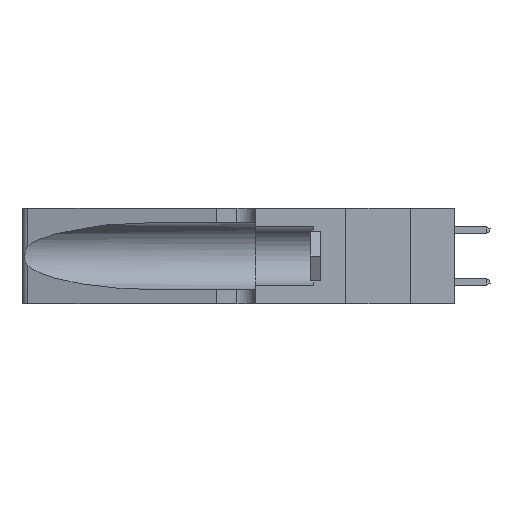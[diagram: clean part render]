
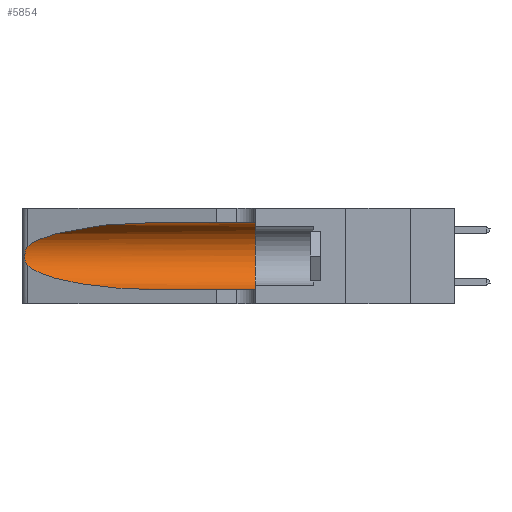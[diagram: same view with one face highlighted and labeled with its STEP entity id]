
A CAD part, left-side view. The second image highlights one B-rep face of the part: STEP entity #5854.
In plain terms, the highlighted cylindrical face has radius 3.308 mm (diameter 6.617 mm), a partial arc.
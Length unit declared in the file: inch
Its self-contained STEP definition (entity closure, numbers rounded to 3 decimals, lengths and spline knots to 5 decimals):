
#1498 = DIRECTION ( 'NONE',  ( 0., 0., -1. ) ) ;
#1572 = DIRECTION ( 'NONE',  ( 0., -1., 0. ) ) ;
#1588 = DIRECTION ( 'NONE',  ( 0., -1., 0. ) ) ;
#1725 = AXIS2_PLACEMENT_3D ( 'NONE', #24249, #1588, #1498 ) ;
#2300 =( BOUNDED_CURVE ( )  B_SPLINE_CURVE ( 3, ( #16898, #26721, #22228, #10949 ),
 .UNSPECIFIED., .F., .T. ) 
 B_SPLINE_CURVE_WITH_KNOTS ( ( 4, 4 ),
 ( 3.44316, 4.71239 ),
 .UNSPECIFIED. ) 
 CURVE ( )  GEOMETRIC_REPRESENTATION_ITEM ( )  RATIONAL_B_SPLINE_CURVE ( ( 1., 0.87, 0.87, 1. ) ) 
 REPRESENTATION_ITEM ( '' )  );
#2474 = CYLINDRICAL_SURFACE ( 'NONE', #1725, 0.13025 ) ;
#4036 = LINE ( 'NONE', #24258, #20734 ) ;
#4125 = CARTESIAN_POINT ( 'NONE',  ( 0.25487, 1.22718, 0.14631 ) ) ;
#4606 = CARTESIAN_POINT ( 'NONE',  ( 0.25639, 1.23184, 0.21858 ) ) ;
#5854 = ADVANCED_FACE ( 'NONE', ( #7828 ), #2474, .F. ) ;
#6089 = CARTESIAN_POINT ( 'NONE',  ( 0.26075, 1.23896, 0.19203 ) ) ;
#6331 = CARTESIAN_POINT ( 'NONE',  ( 0.26075, 1.23896, 0.178 ) ) ;
#7218 = CARTESIAN_POINT ( 'NONE',  ( 0.1305, 0.35, 0.185 ) ) ;
#7424 = ORIENTED_EDGE ( 'NONE', *, *, #10110, .T. ) ;
#7828 = FACE_OUTER_BOUND ( 'NONE', #10877, .T. ) ;
#8082 = EDGE_CURVE ( 'NONE', #15675, #22160, #2300, .T. ) ;
#8282 = CARTESIAN_POINT ( 'NONE',  ( 0.25854, 1.2359, 0.20912 ) ) ;
#8344 = CARTESIAN_POINT ( 'NONE',  ( 0.1305, 1.61858, 0.05475 ) ) ;
#9031 = CARTESIAN_POINT ( 'NONE',  ( 0.1305, 0.72297, 0.31525 ) ) ;
#10110 = EDGE_CURVE ( 'NONE', #22160, #10908, #26794, .T. ) ;
#10643 = CARTESIAN_POINT ( 'NONE',  ( 0.2373, 1.15595, 0.28018 ) ) ;
#10764 = VERTEX_POINT ( 'NONE', #26175 ) ;
#10877 = EDGE_LOOP ( 'NONE', ( #24536, #21921, #24334, #7424, #19852, #14446 ) ) ;
#10908 = VERTEX_POINT ( 'NONE', #22279 ) ;
#10949 = CARTESIAN_POINT ( 'NONE',  ( 0.1305, 0.72297, 0.05475 ) ) ;
#11233 = CARTESIAN_POINT ( 'NONE',  ( 0.25787, 1.23484, 0.2124 ) ) ;
#11376 = EDGE_CURVE ( 'NONE', #24390, #26412, #4036, .T. ) ;
#12306 = CARTESIAN_POINT ( 'NONE',  ( 0.25487, 1.22718, 0.22369 ) ) ;
#13304 = CARTESIAN_POINT ( 'NONE',  ( 0.25639, 1.23186, 0.15144 ) ) ;
#14188 = CIRCLE ( 'NONE', #24427, 0.13025 ) ;
#14346 = CARTESIAN_POINT ( 'NONE',  ( 0.25555, 1.22994, 0.2215 ) ) ;
#14396 = CARTESIAN_POINT ( 'NONE',  ( 0.26018, 1.23835, 0.19895 ) ) ;
#14424 = EDGE_CURVE ( 'NONE', #26412, #10908, #14188, .T. ) ;
#14446 = ORIENTED_EDGE ( 'NONE', *, *, #11376, .F. ) ;
#14663 = CARTESIAN_POINT ( 'NONE',  ( 0.25487, 1.22718, 0.14631 ) ) ;
#15481 = CARTESIAN_POINT ( 'NONE',  ( 0.26017, 1.23833, 0.17102 ) ) ;
#15489 = CARTESIAN_POINT ( 'NONE',  ( 0.1305, 0.72297, 0.05475 ) ) ;
#15575 = CARTESIAN_POINT ( 'NONE',  ( 0.25555, 1.22993, 0.14849 ) ) ;
#15675 = VERTEX_POINT ( 'NONE', #14663 ) ;
#15971 = EDGE_CURVE ( 'NONE', #10764, #15675, #27092, .T. ) ;
#16898 = CARTESIAN_POINT ( 'NONE',  ( 0.25487, 1.22718, 0.14631 ) ) ;
#17642 = CARTESIAN_POINT ( 'NONE',  ( 0.1305, 0.35, 0.31525 ) ) ;
#17746 = CARTESIAN_POINT ( 'NONE',  ( 0.25856, 1.23593, 0.16098 ) ) ;
#18058 = CARTESIAN_POINT ( 'NONE',  ( 0.18966, 0.96281, 0.31525 ) ) ;
#19852 = ORIENTED_EDGE ( 'NONE', *, *, #14424, .F. ) ;
#20734 = VECTOR ( 'NONE', #21660, 39.37008 ) ;
#20750 = VECTOR ( 'NONE', #1572, 39.37008 ) ;
#20777 = EDGE_CURVE ( 'NONE', #24390, #10764, #21792, .T. ) ;
#21096 = DIRECTION ( 'NONE',  ( 0., 0., 1. ) ) ;
#21660 = DIRECTION ( 'NONE',  ( 0., -1., 0. ) ) ;
#21792 =( BOUNDED_CURVE ( )  B_SPLINE_CURVE ( 3, ( #9031, #18058, #10643, #22311 ),
 .UNSPECIFIED., .F., .T. ) 
 B_SPLINE_CURVE_WITH_KNOTS ( ( 4, 4 ),
 ( 1.5708, 2.84003 ),
 .UNSPECIFIED. ) 
 CURVE ( )  GEOMETRIC_REPRESENTATION_ITEM ( )  RATIONAL_B_SPLINE_CURVE ( ( 1., 0.87, 0.87, 1. ) ) 
 REPRESENTATION_ITEM ( '' )  );
#21921 = ORIENTED_EDGE ( 'NONE', *, *, #15971, .T. ) ;
#22160 = VERTEX_POINT ( 'NONE', #15489 ) ;
#22228 = CARTESIAN_POINT ( 'NONE',  ( 0.18966, 0.96281, 0.05475 ) ) ;
#22279 = CARTESIAN_POINT ( 'NONE',  ( 0.1305, 0.35, 0.05475 ) ) ;
#22311 = CARTESIAN_POINT ( 'NONE',  ( 0.25487, 1.22718, 0.22369 ) ) ;
#22579 = CARTESIAN_POINT ( 'NONE',  ( 0.1305, 0.72297, 0.31525 ) ) ;
#24249 = CARTESIAN_POINT ( 'NONE',  ( 0.1305, 1.61858, 0.185 ) ) ;
#24258 = CARTESIAN_POINT ( 'NONE',  ( 0.1305, 1.61858, 0.31525 ) ) ;
#24334 = ORIENTED_EDGE ( 'NONE', *, *, #8082, .T. ) ;
#24390 = VERTEX_POINT ( 'NONE', #22579 ) ;
#24427 = AXIS2_PLACEMENT_3D ( 'NONE', #7218, #26454, #21096 ) ;
#24536 = ORIENTED_EDGE ( 'NONE', *, *, #20777, .T. ) ;
#24591 = CARTESIAN_POINT ( 'NONE',  ( 0.25789, 1.23486, 0.15765 ) ) ;
#26175 = CARTESIAN_POINT ( 'NONE',  ( 0.25487, 1.22718, 0.22369 ) ) ;
#26412 = VERTEX_POINT ( 'NONE', #17642 ) ;
#26454 = DIRECTION ( 'NONE',  ( 0., 1., 0. ) ) ;
#26721 = CARTESIAN_POINT ( 'NONE',  ( 0.2373, 1.15595, 0.08982 ) ) ;
#26794 = LINE ( 'NONE', #8344, #20750 ) ;
#27092 = B_SPLINE_CURVE_WITH_KNOTS ( 'NONE', 3,
 ( #12306, #14346, #4606, #11233, #8282, #14396, #6089, #6331, #15481, #17746, #24591, #13304, #15575, #4125 ),
 .UNSPECIFIED., .F., .F.,
 ( 4, 2, 2, 2, 2, 2, 4 ),
 ( 0., 0.00027, 0.00053, 0.00107, 0.0016, 0.00187, 0.00214 ),
 .UNSPECIFIED. ) ;
